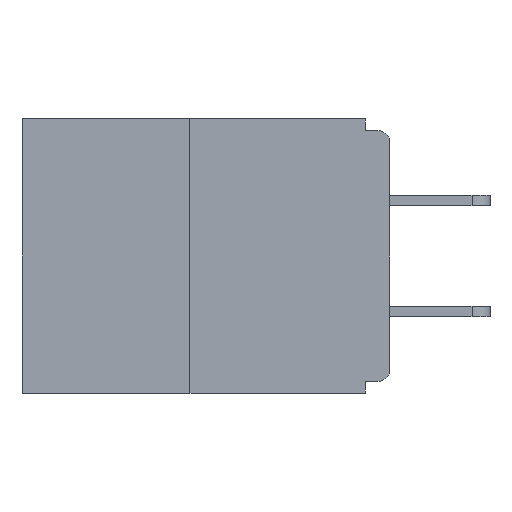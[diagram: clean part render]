
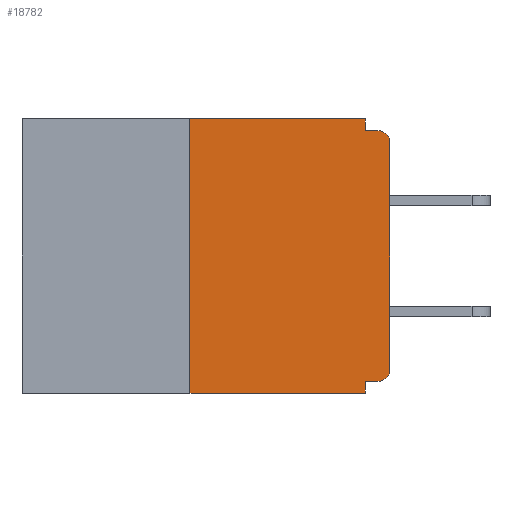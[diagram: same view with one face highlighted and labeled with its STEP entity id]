
A CAD part, left-side view. The second image highlights one B-rep face of the part: STEP entity #18782.
In plain terms, the highlighted planar face has unit normal (-1, 0, 0).
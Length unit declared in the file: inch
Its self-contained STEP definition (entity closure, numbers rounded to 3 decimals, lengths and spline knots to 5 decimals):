
#371 = DIRECTION ( 'NONE',  ( 0., -1., 0. ) ) ;
#1053 = LINE ( 'NONE', #18934, #24309 ) ;
#1207 = LINE ( 'NONE', #4760, #15954 ) ;
#1483 = DIRECTION ( 'NONE',  ( 0., 0., -1. ) ) ;
#2010 = AXIS2_PLACEMENT_3D ( 'NONE', #4627, #20332, #6876 ) ;
#2021 = ORIENTED_EDGE ( 'NONE', *, *, #28836, .F. ) ;
#2202 = ORIENTED_EDGE ( 'NONE', *, *, #11694, .T. ) ;
#2360 = VERTEX_POINT ( 'NONE', #28027 ) ;
#2621 = EDGE_CURVE ( 'NONE', #23147, #13584, #5871, .T. ) ;
#3291 = DIRECTION ( 'NONE',  ( 0., 0., 1. ) ) ;
#3714 = CARTESIAN_POINT ( 'NONE',  ( 0., 0.015, -0.03 ) ) ;
#3950 = VERTEX_POINT ( 'NONE', #7746 ) ;
#4111 = VERTEX_POINT ( 'NONE', #28041 ) ;
#4223 = CARTESIAN_POINT ( 'NONE',  ( 0., 0., -0.313 ) ) ;
#4448 = EDGE_CURVE ( 'NONE', #28097, #21810, #5388, .T. ) ;
#4609 = LINE ( 'NONE', #24219, #24240 ) ;
#4627 = CARTESIAN_POINT ( 'NONE',  ( 0., 0.46, 0. ) ) ;
#4760 = CARTESIAN_POINT ( 'NONE',  ( 0., 0.46, -0.343 ) ) ;
#5388 = LINE ( 'NONE', #22651, #16970 ) ;
#5807 = DIRECTION ( 'NONE',  ( 0., 0., 1. ) ) ;
#5871 = LINE ( 'NONE', #26841, #16417 ) ;
#6376 = ORIENTED_EDGE ( 'NONE', *, *, #2621, .F. ) ;
#6489 = ORIENTED_EDGE ( 'NONE', *, *, #25506, .T. ) ;
#6499 = PLANE ( 'NONE',  #2010 ) ;
#6845 = DIRECTION ( 'NONE',  ( -1., 0., 0. ) ) ;
#6876 = DIRECTION ( 'NONE',  ( 0., 0., -1. ) ) ;
#6912 = AXIS2_PLACEMENT_3D ( 'NONE', #28412, #26265, #8324 ) ;
#7017 = CIRCLE ( 'NONE', #22412, 0.015 ) ;
#7068 = CARTESIAN_POINT ( 'NONE',  ( 0., 0.015, -0.328 ) ) ;
#7746 = CARTESIAN_POINT ( 'NONE',  ( 0., 0.031, -0.343 ) ) ;
#7857 = CARTESIAN_POINT ( 'NONE',  ( 0., 0.25, 0. ) ) ;
#8324 = DIRECTION ( 'NONE',  ( 0., 0., -1. ) ) ;
#9646 = VECTOR ( 'NONE', #5807, 39.37008 ) ;
#10090 = DIRECTION ( 'NONE',  ( 0., -1., 0. ) ) ;
#10271 = VECTOR ( 'NONE', #3291, 39.37008 ) ;
#10559 = LINE ( 'NONE', #25572, #26344 ) ;
#10614 = DIRECTION ( 'NONE',  ( 0., 0., -1. ) ) ;
#11694 = EDGE_CURVE ( 'NONE', #23147, #17285, #19031, .T. ) ;
#12643 = ORIENTED_EDGE ( 'NONE', *, *, #13795, .F. ) ;
#13158 = EDGE_LOOP ( 'NONE', ( #12643, #2021, #23237, #24827, #6376, #2202, #28539, #6489, #28333, #19064 ) ) ;
#13584 = VERTEX_POINT ( 'NONE', #27389 ) ;
#13795 = EDGE_CURVE ( 'NONE', #4111, #2360, #1053, .T. ) ;
#13799 = FACE_OUTER_BOUND ( 'NONE', #13158, .T. ) ;
#15518 = CARTESIAN_POINT ( 'NONE',  ( 0., 0., -0.03 ) ) ;
#15665 = LINE ( 'NONE', #7857, #9646 ) ;
#15954 = VECTOR ( 'NONE', #371, 39.37008 ) ;
#16417 = VECTOR ( 'NONE', #22248, 39.37008 ) ;
#16572 = VERTEX_POINT ( 'NONE', #19024 ) ;
#16970 = VECTOR ( 'NONE', #24964, 39.37008 ) ;
#17285 = VERTEX_POINT ( 'NONE', #4223 ) ;
#18237 = EDGE_CURVE ( 'NONE', #16572, #3950, #1207, .T. ) ;
#18782 = ADVANCED_FACE ( 'NONE', ( #13799 ), #6499, .F. ) ;
#18934 = CARTESIAN_POINT ( 'NONE',  ( 0., 0.46, 0. ) ) ;
#19024 = CARTESIAN_POINT ( 'NONE',  ( 0., 0.25, -0.343 ) ) ;
#19031 = CIRCLE ( 'NONE', #6912, 0.015 ) ;
#19064 = ORIENTED_EDGE ( 'NONE', *, *, #25217, .F. ) ;
#19435 = CARTESIAN_POINT ( 'NONE',  ( 0., 0.031, -0.015 ) ) ;
#20332 = DIRECTION ( 'NONE',  ( 1., 0., 0. ) ) ;
#20401 = CARTESIAN_POINT ( 'NONE',  ( 0., 0.015, -0.015 ) ) ;
#20960 = CARTESIAN_POINT ( 'NONE',  ( 0., 0., 0. ) ) ;
#21189 = DIRECTION ( 'NONE',  ( 0., 0., -1. ) ) ;
#21810 = VERTEX_POINT ( 'NONE', #20401 ) ;
#21859 = VERTEX_POINT ( 'NONE', #15518 ) ;
#22248 = DIRECTION ( 'NONE',  ( 0., 1., 0. ) ) ;
#22412 = AXIS2_PLACEMENT_3D ( 'NONE', #3714, #6845, #10614 ) ;
#22651 = CARTESIAN_POINT ( 'NONE',  ( 0., 0., -0.015 ) ) ;
#23147 = VERTEX_POINT ( 'NONE', #7068 ) ;
#23237 = ORIENTED_EDGE ( 'NONE', *, *, #18237, .T. ) ;
#23265 = LINE ( 'NONE', #20960, #10271 ) ;
#23938 = EDGE_CURVE ( 'NONE', #17285, #21859, #23265, .T. ) ;
#24219 = CARTESIAN_POINT ( 'NONE',  ( 0., 0.031, 0. ) ) ;
#24240 = VECTOR ( 'NONE', #1483, 39.37008 ) ;
#24309 = VECTOR ( 'NONE', #10090, 39.37008 ) ;
#24827 = ORIENTED_EDGE ( 'NONE', *, *, #25109, .F. ) ;
#24964 = DIRECTION ( 'NONE',  ( 0., -1., 0. ) ) ;
#25109 = EDGE_CURVE ( 'NONE', #13584, #3950, #10559, .T. ) ;
#25217 = EDGE_CURVE ( 'NONE', #2360, #28097, #4609, .T. ) ;
#25506 = EDGE_CURVE ( 'NONE', #21859, #21810, #7017, .T. ) ;
#25572 = CARTESIAN_POINT ( 'NONE',  ( 0., 0.031, -0.343 ) ) ;
#26265 = DIRECTION ( 'NONE',  ( -1., 0., 0. ) ) ;
#26344 = VECTOR ( 'NONE', #21189, 39.37008 ) ;
#26841 = CARTESIAN_POINT ( 'NONE',  ( 0., 0., -0.328 ) ) ;
#27389 = CARTESIAN_POINT ( 'NONE',  ( 0., 0.031, -0.328 ) ) ;
#28027 = CARTESIAN_POINT ( 'NONE',  ( 0., 0.031, 0. ) ) ;
#28041 = CARTESIAN_POINT ( 'NONE',  ( 0., 0.25, 0. ) ) ;
#28097 = VERTEX_POINT ( 'NONE', #19435 ) ;
#28333 = ORIENTED_EDGE ( 'NONE', *, *, #4448, .F. ) ;
#28412 = CARTESIAN_POINT ( 'NONE',  ( 0., 0.015, -0.313 ) ) ;
#28539 = ORIENTED_EDGE ( 'NONE', *, *, #23938, .T. ) ;
#28836 = EDGE_CURVE ( 'NONE', #16572, #4111, #15665, .T. ) ;
